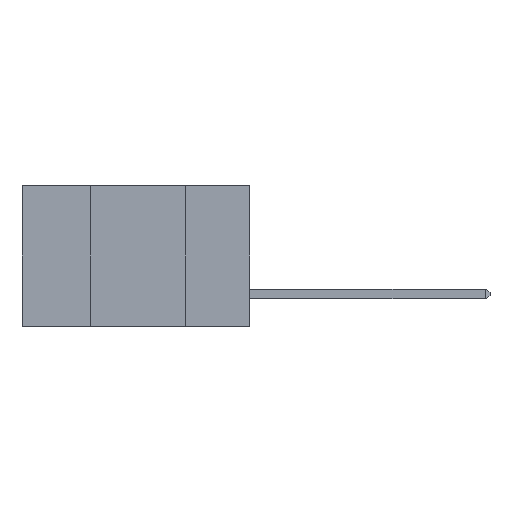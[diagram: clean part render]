
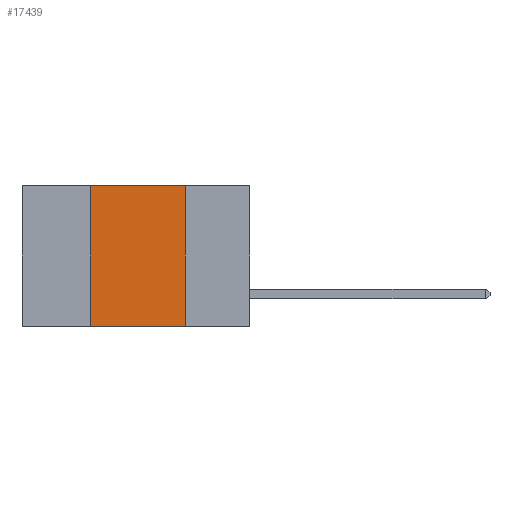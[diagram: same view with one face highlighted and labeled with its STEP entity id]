
A CAD part, left-side view. The second image highlights one B-rep face of the part: STEP entity #17439.
In plain terms, the highlighted planar face has unit normal (-1, 0, 0).
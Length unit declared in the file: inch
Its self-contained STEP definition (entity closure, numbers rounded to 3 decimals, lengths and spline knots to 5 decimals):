
#855 = CARTESIAN_POINT ( 'NONE',  ( 0., 0.6, -0.37 ) ) ;
#988 = DIRECTION ( 'NONE',  ( 0., 0., -1. ) ) ;
#1350 = VECTOR ( 'NONE', #8882, 39.37008 ) ;
#2228 = FACE_OUTER_BOUND ( 'NONE', #23435, .T. ) ;
#2926 = EDGE_CURVE ( 'NONE', #8693, #24177, #18707, .T. ) ;
#2948 = VECTOR ( 'NONE', #988, 39.37008 ) ;
#3812 = ORIENTED_EDGE ( 'NONE', *, *, #3926, .F. ) ;
#3926 = EDGE_CURVE ( 'NONE', #13418, #6953, #5152, .T. ) ;
#4537 = VECTOR ( 'NONE', #18233, 39.37008 ) ;
#4893 = CARTESIAN_POINT ( 'NONE',  ( 0., 0.42, -0.37 ) ) ;
#5152 = LINE ( 'NONE', #24047, #4537 ) ;
#6953 = VERTEX_POINT ( 'NONE', #23039 ) ;
#7015 = CARTESIAN_POINT ( 'NONE',  ( 0., 0.17, 0. ) ) ;
#7569 = ORIENTED_EDGE ( 'NONE', *, *, #2926, .F. ) ;
#7830 = LINE ( 'NONE', #18741, #22252 ) ;
#7940 = CARTESIAN_POINT ( 'NONE',  ( 0., 0.6, 0. ) ) ;
#8693 = VERTEX_POINT ( 'NONE', #7015 ) ;
#8882 = DIRECTION ( 'NONE',  ( 0., -1., 0. ) ) ;
#10975 = ORIENTED_EDGE ( 'NONE', *, *, #17689, .F. ) ;
#11927 = PLANE ( 'NONE',  #16653 ) ;
#13418 = VERTEX_POINT ( 'NONE', #4893 ) ;
#13922 = DIRECTION ( 'NONE',  ( 0., 0., -1. ) ) ;
#15228 = CARTESIAN_POINT ( 'NONE',  ( 0., 0.17, -0.37 ) ) ;
#16653 = AXIS2_PLACEMENT_3D ( 'NONE', #7940, #20276, #13922 ) ;
#17127 = LINE ( 'NONE', #855, #1350 ) ;
#17439 = ADVANCED_FACE ( 'NONE', ( #2228 ), #11927, .F. ) ;
#17689 = EDGE_CURVE ( 'NONE', #6953, #8693, #7830, .T. ) ;
#18233 = DIRECTION ( 'NONE',  ( 0., 0., 1. ) ) ;
#18707 = LINE ( 'NONE', #24573, #2948 ) ;
#18741 = CARTESIAN_POINT ( 'NONE',  ( 0., 0.6, 0. ) ) ;
#20276 = DIRECTION ( 'NONE',  ( 1., 0., 0. ) ) ;
#22080 = EDGE_CURVE ( 'NONE', #13418, #24177, #17127, .T. ) ;
#22252 = VECTOR ( 'NONE', #24619, 39.37008 ) ;
#23039 = CARTESIAN_POINT ( 'NONE',  ( 0., 0.42, 0. ) ) ;
#23435 = EDGE_LOOP ( 'NONE', ( #7569, #10975, #3812, #25354 ) ) ;
#24047 = CARTESIAN_POINT ( 'NONE',  ( 0., 0.42, 0. ) ) ;
#24177 = VERTEX_POINT ( 'NONE', #15228 ) ;
#24573 = CARTESIAN_POINT ( 'NONE',  ( 0., 0.17, 0. ) ) ;
#24619 = DIRECTION ( 'NONE',  ( 0., -1., 0. ) ) ;
#25354 = ORIENTED_EDGE ( 'NONE', *, *, #22080, .T. ) ;
